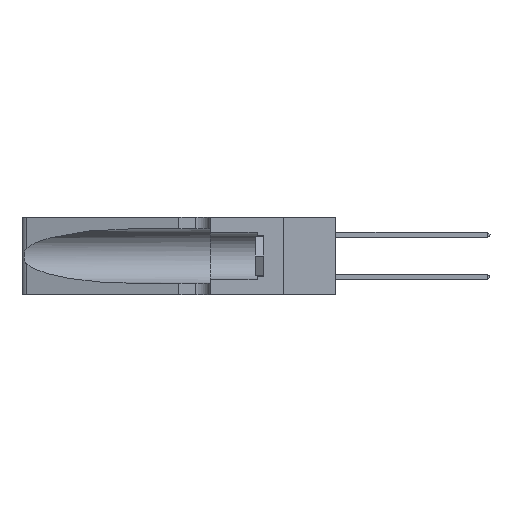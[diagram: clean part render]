
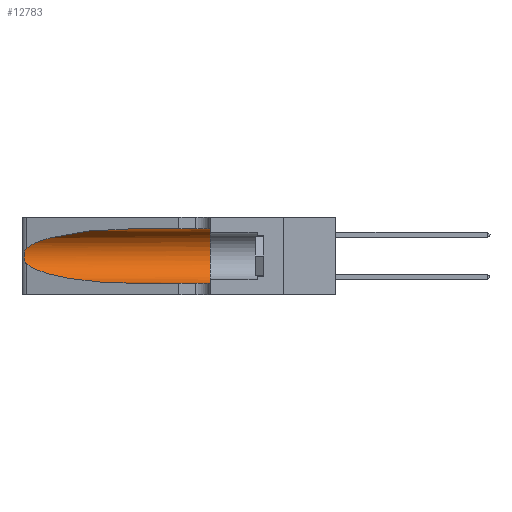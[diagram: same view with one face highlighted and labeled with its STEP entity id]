
A CAD part, left-side view. The second image highlights one B-rep face of the part: STEP entity #12783.
In plain terms, the highlighted cylindrical face has radius 3.308 mm (diameter 6.617 mm), a partial arc.
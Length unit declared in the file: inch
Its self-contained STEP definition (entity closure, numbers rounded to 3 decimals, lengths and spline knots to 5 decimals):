
#1574 = CARTESIAN_POINT ( 'NONE',  ( 0.1305, 0.72297, 0.05475 ) ) ;
#2413 =( BOUNDED_CURVE ( )  B_SPLINE_CURVE ( 3, ( #3427, #13767, #22208, #23692 ),
 .UNSPECIFIED., .F., .F. ) 
 B_SPLINE_CURVE_WITH_KNOTS ( ( 4, 4 ),
 ( 3.44316, 4.71239 ),
 .UNSPECIFIED. ) 
 CURVE ( )  GEOMETRIC_REPRESENTATION_ITEM ( )  RATIONAL_B_SPLINE_CURVE ( ( 1., 0.87, 0.87, 1. ) ) 
 REPRESENTATION_ITEM ( '' )  );
#3133 = AXIS2_PLACEMENT_3D ( 'NONE', #3588, #10137, #18601 ) ;
#3210 = VERTEX_POINT ( 'NONE', #9568 ) ;
#3427 = CARTESIAN_POINT ( 'NONE',  ( 0.25487, 1.22718, 0.14631 ) ) ;
#3588 = CARTESIAN_POINT ( 'NONE',  ( 0.1305, 1.61858, 0.185 ) ) ;
#4187 = ORIENTED_EDGE ( 'NONE', *, *, #8830, .T. ) ;
#4425 = CARTESIAN_POINT ( 'NONE',  ( 0.25487, 1.22718, 0.22369 ) ) ;
#4721 = ORIENTED_EDGE ( 'NONE', *, *, #15276, .F. ) ;
#5135 = CARTESIAN_POINT ( 'NONE',  ( 0.26018, 1.23835, 0.19895 ) ) ;
#5359 = VERTEX_POINT ( 'NONE', #21979 ) ;
#5472 = CARTESIAN_POINT ( 'NONE',  ( 0.1305, 0.35, 0.185 ) ) ;
#5616 = B_SPLINE_CURVE_WITH_KNOTS ( 'NONE', 3,
 ( #13864, #20190, #22291, #9692, #24362, #5135, #19825, #7215, #23085, #17237, #23603, #7568, #26142, #15703 ),
 .UNSPECIFIED., .F., .F.,
 ( 4, 2, 2, 2, 2, 2, 4 ),
 ( 0., 0.00027, 0.00053, 0.00107, 0.0016, 0.00187, 0.00214 ),
 .UNSPECIFIED. ) ;
#6441 = CARTESIAN_POINT ( 'NONE',  ( 0.2373, 1.15595, 0.28018 ) ) ;
#6770 = VERTEX_POINT ( 'NONE', #1574 ) ;
#7215 = CARTESIAN_POINT ( 'NONE',  ( 0.26075, 1.23896, 0.178 ) ) ;
#7568 = CARTESIAN_POINT ( 'NONE',  ( 0.25639, 1.23186, 0.15144 ) ) ;
#7660 = DIRECTION ( 'NONE',  ( 0., 1., 0. ) ) ;
#8617 = VECTOR ( 'NONE', #9464, 39.37008 ) ;
#8830 = EDGE_CURVE ( 'NONE', #6770, #25915, #23350, .T. ) ;
#8978 = VERTEX_POINT ( 'NONE', #16117 ) ;
#9464 = DIRECTION ( 'NONE',  ( 0., -1., 0. ) ) ;
#9568 = CARTESIAN_POINT ( 'NONE',  ( 0.1305, 0.72297, 0.31525 ) ) ;
#9692 = CARTESIAN_POINT ( 'NONE',  ( 0.25787, 1.23484, 0.2124 ) ) ;
#10137 = DIRECTION ( 'NONE',  ( 0., -1., 0. ) ) ;
#10571 = CARTESIAN_POINT ( 'NONE',  ( 0.18966, 0.96281, 0.31525 ) ) ;
#11366 = EDGE_CURVE ( 'NONE', #3210, #23994, #20624, .T. ) ;
#12100 = CARTESIAN_POINT ( 'NONE',  ( 0.1305, 1.61858, 0.31525 ) ) ;
#12474 = EDGE_CURVE ( 'NONE', #5359, #8978, #5616, .T. ) ;
#12783 = ADVANCED_FACE ( 'NONE', ( #15273 ), #14646, .F. ) ;
#13767 = CARTESIAN_POINT ( 'NONE',  ( 0.2373, 1.15595, 0.08982 ) ) ;
#13864 = CARTESIAN_POINT ( 'NONE',  ( 0.25487, 1.22718, 0.22369 ) ) ;
#14142 = AXIS2_PLACEMENT_3D ( 'NONE', #5472, #7660, #22361 ) ;
#14646 = CYLINDRICAL_SURFACE ( 'NONE', #3133, 0.13025 ) ;
#15256 = ORIENTED_EDGE ( 'NONE', *, *, #17138, .T. ) ;
#15273 = FACE_OUTER_BOUND ( 'NONE', #18968, .T. ) ;
#15276 = EDGE_CURVE ( 'NONE', #23994, #25915, #17064, .T. ) ;
#15703 = CARTESIAN_POINT ( 'NONE',  ( 0.25487, 1.22718, 0.14631 ) ) ;
#15765 = EDGE_CURVE ( 'NONE', #8978, #6770, #2413, .T. ) ;
#16117 = CARTESIAN_POINT ( 'NONE',  ( 0.25487, 1.22718, 0.14631 ) ) ;
#17064 = CIRCLE ( 'NONE', #14142, 0.13025 ) ;
#17138 = EDGE_CURVE ( 'NONE', #3210, #5359, #24752, .T. ) ;
#17237 = CARTESIAN_POINT ( 'NONE',  ( 0.25856, 1.23593, 0.16098 ) ) ;
#17846 = ORIENTED_EDGE ( 'NONE', *, *, #12474, .T. ) ;
#17880 = CARTESIAN_POINT ( 'NONE',  ( 0.1305, 0.35, 0.05475 ) ) ;
#18086 = ORIENTED_EDGE ( 'NONE', *, *, #11366, .F. ) ;
#18601 = DIRECTION ( 'NONE',  ( 0., 0., -1. ) ) ;
#18873 = CARTESIAN_POINT ( 'NONE',  ( 0.1305, 1.61858, 0.05475 ) ) ;
#18968 = EDGE_LOOP ( 'NONE', ( #15256, #17846, #22269, #4187, #4721, #18086 ) ) ;
#19825 = CARTESIAN_POINT ( 'NONE',  ( 0.26075, 1.23896, 0.19203 ) ) ;
#19959 = CARTESIAN_POINT ( 'NONE',  ( 0.1305, 0.35, 0.31525 ) ) ;
#20190 = CARTESIAN_POINT ( 'NONE',  ( 0.25555, 1.22994, 0.2215 ) ) ;
#20624 = LINE ( 'NONE', #12100, #21611 ) ;
#21611 = VECTOR ( 'NONE', #24544, 39.37008 ) ;
#21979 = CARTESIAN_POINT ( 'NONE',  ( 0.25487, 1.22718, 0.22369 ) ) ;
#22208 = CARTESIAN_POINT ( 'NONE',  ( 0.18966, 0.96281, 0.05475 ) ) ;
#22269 = ORIENTED_EDGE ( 'NONE', *, *, #15765, .T. ) ;
#22291 = CARTESIAN_POINT ( 'NONE',  ( 0.25639, 1.23184, 0.21858 ) ) ;
#22361 = DIRECTION ( 'NONE',  ( 0., 0., 1. ) ) ;
#23085 = CARTESIAN_POINT ( 'NONE',  ( 0.26017, 1.23833, 0.17102 ) ) ;
#23350 = LINE ( 'NONE', #18873, #8617 ) ;
#23603 = CARTESIAN_POINT ( 'NONE',  ( 0.25789, 1.23486, 0.15765 ) ) ;
#23692 = CARTESIAN_POINT ( 'NONE',  ( 0.1305, 0.72297, 0.05475 ) ) ;
#23994 = VERTEX_POINT ( 'NONE', #19959 ) ;
#24362 = CARTESIAN_POINT ( 'NONE',  ( 0.25854, 1.2359, 0.20912 ) ) ;
#24544 = DIRECTION ( 'NONE',  ( 0., -1., 0. ) ) ;
#24752 =( BOUNDED_CURVE ( )  B_SPLINE_CURVE ( 3, ( #25598, #10571, #6441, #4425 ),
 .UNSPECIFIED., .F., .T. ) 
 B_SPLINE_CURVE_WITH_KNOTS ( ( 4, 4 ),
 ( 1.5708, 2.84003 ),
 .UNSPECIFIED. ) 
 CURVE ( )  GEOMETRIC_REPRESENTATION_ITEM ( )  RATIONAL_B_SPLINE_CURVE ( ( 1., 0.87, 0.87, 1. ) ) 
 REPRESENTATION_ITEM ( '' )  );
#25598 = CARTESIAN_POINT ( 'NONE',  ( 0.1305, 0.72297, 0.31525 ) ) ;
#25915 = VERTEX_POINT ( 'NONE', #17880 ) ;
#26142 = CARTESIAN_POINT ( 'NONE',  ( 0.25555, 1.22993, 0.14849 ) ) ;
